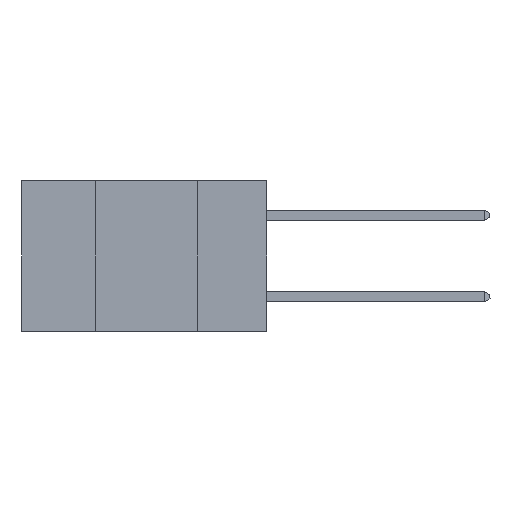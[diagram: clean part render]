
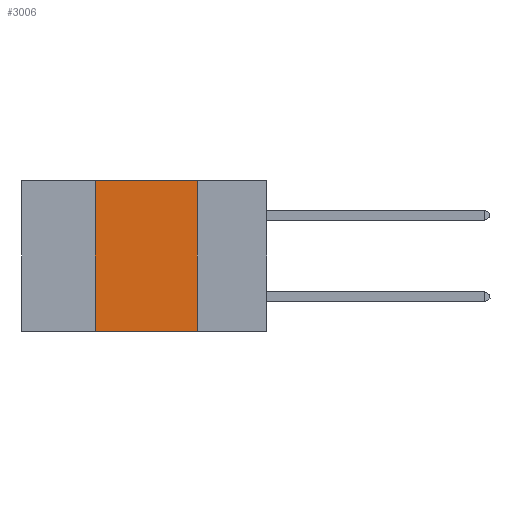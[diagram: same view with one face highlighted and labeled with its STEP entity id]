
A CAD part, left-side view. The second image highlights one B-rep face of the part: STEP entity #3006.
In plain terms, the highlighted planar face has unit normal (-1, 0, 0).
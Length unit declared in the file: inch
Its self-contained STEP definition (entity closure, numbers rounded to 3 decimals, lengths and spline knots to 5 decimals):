
#268 = ORIENTED_EDGE ( 'NONE', *, *, #22263, .F. ) ;
#1234 = LINE ( 'NONE', #21088, #14165 ) ;
#1333 = DIRECTION ( 'NONE',  ( 1., 0., 0. ) ) ;
#1346 = LINE ( 'NONE', #6564, #6185 ) ;
#1625 = VERTEX_POINT ( 'NONE', #6363 ) ;
#2627 = LINE ( 'NONE', #6499, #11512 ) ;
#2915 = ORIENTED_EDGE ( 'NONE', *, *, #19989, .T. ) ;
#3006 = ADVANCED_FACE ( 'NONE', ( #11524 ), #11973, .F. ) ;
#3208 = EDGE_CURVE ( 'NONE', #22579, #4501, #1234, .T. ) ;
#3450 = DIRECTION ( 'NONE',  ( 0., -1., 0. ) ) ;
#4501 = VERTEX_POINT ( 'NONE', #9083 ) ;
#4511 = AXIS2_PLACEMENT_3D ( 'NONE', #10236, #1333, #13684 ) ;
#5876 = VECTOR ( 'NONE', #3450, 39.37008 ) ;
#6185 = VECTOR ( 'NONE', #16893, 39.37008 ) ;
#6363 = CARTESIAN_POINT ( 'NONE',  ( 0., 0.42, -0.37 ) ) ;
#6379 = VERTEX_POINT ( 'NONE', #18253 ) ;
#6499 = CARTESIAN_POINT ( 'NONE',  ( 0., 0.42, 0. ) ) ;
#6564 = CARTESIAN_POINT ( 'NONE',  ( 0., 0.6, -0.37 ) ) ;
#9083 = CARTESIAN_POINT ( 'NONE',  ( 0., 0.17, -0.37 ) ) ;
#10236 = CARTESIAN_POINT ( 'NONE',  ( 0., 0.6, 0. ) ) ;
#10521 = LINE ( 'NONE', #22479, #5876 ) ;
#11512 = VECTOR ( 'NONE', #20311, 39.37008 ) ;
#11524 = FACE_OUTER_BOUND ( 'NONE', #15352, .T. ) ;
#11973 = PLANE ( 'NONE',  #4511 ) ;
#13684 = DIRECTION ( 'NONE',  ( 0., 0., -1. ) ) ;
#14165 = VECTOR ( 'NONE', #19339, 39.37008 ) ;
#14259 = CARTESIAN_POINT ( 'NONE',  ( 0., 0.17, 0. ) ) ;
#15352 = EDGE_LOOP ( 'NONE', ( #20746, #21034, #268, #2915 ) ) ;
#16893 = DIRECTION ( 'NONE',  ( 0., -1., 0. ) ) ;
#18253 = CARTESIAN_POINT ( 'NONE',  ( 0., 0.42, 0. ) ) ;
#19339 = DIRECTION ( 'NONE',  ( 0., 0., -1. ) ) ;
#19989 = EDGE_CURVE ( 'NONE', #1625, #4501, #1346, .T. ) ;
#20311 = DIRECTION ( 'NONE',  ( 0., 0., 1. ) ) ;
#20660 = EDGE_CURVE ( 'NONE', #6379, #22579, #10521, .T. ) ;
#20746 = ORIENTED_EDGE ( 'NONE', *, *, #3208, .F. ) ;
#21034 = ORIENTED_EDGE ( 'NONE', *, *, #20660, .F. ) ;
#21088 = CARTESIAN_POINT ( 'NONE',  ( 0., 0.17, 0. ) ) ;
#22263 = EDGE_CURVE ( 'NONE', #1625, #6379, #2627, .T. ) ;
#22479 = CARTESIAN_POINT ( 'NONE',  ( 0., 0.6, 0. ) ) ;
#22579 = VERTEX_POINT ( 'NONE', #14259 ) ;
